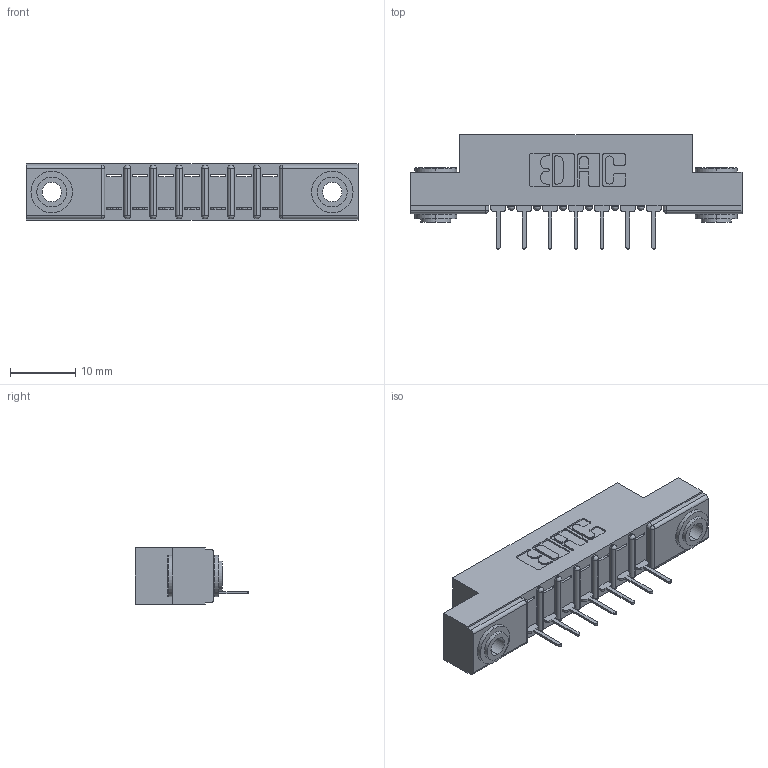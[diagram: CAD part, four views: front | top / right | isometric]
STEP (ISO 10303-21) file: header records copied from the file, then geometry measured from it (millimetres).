
FILE_DESCRIPTION (( 'STEP AP203' ), '1' );
FILE_NAME ('307-007-531-103.STEP', '2019-09-03T13:50:21', ( '' ), ( '' ), 'SwSTEP 2.0', 'SolidWorks 2016', '' );
FILE_SCHEMA (( 'CONFIG_CONTROL_DESIGN' ));
Length unit declared in the file: inch
Products named in the file (4): 345-250-002_345-250-002-102; 307 Part_.156 Dia Mounting Holes; 307-007-531-103; 307-290-001_531
Assembly tree (10 placements, depth 2):
  307-007-531-103
    307 Part_.156 Dia Mounting Holes
    307-290-001_531  x7
    345-250-002_345-250-002-102  x2
Bounding box: 50.75 x 17.42 x 8.71 mm (x, y, z)
Volume: 3229.9 mm3; surface area: 4624.9 mm2
Topology: 10 solids, 10 shells, 570 faces, 1569 edges, 1010 vertices
Faces by surface type: plane 353, cylinder 193, sphere 16, cone 8
Entity records: 11349 total; most frequent: CARTESIAN_POINT 1877, DIRECTION 1861, ORIENTED_EDGE 1854, EDGE_CURVE 927, LINE 689, VECTOR 689, VERTEX_POINT 602, AXIS2_PLACEMENT_3D 586
